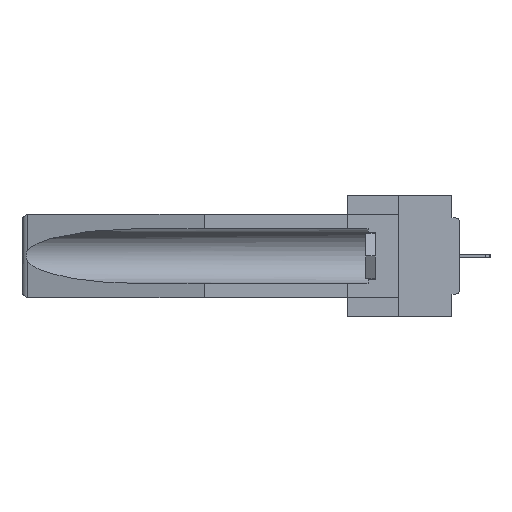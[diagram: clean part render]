
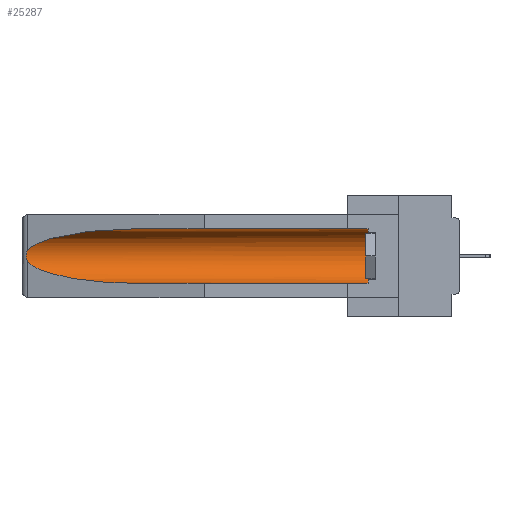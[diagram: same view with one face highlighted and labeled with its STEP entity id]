
A CAD part, left-side view. The second image highlights one B-rep face of the part: STEP entity #25287.
In plain terms, the highlighted cylindrical face has radius 2.857 mm (diameter 5.715 mm), a partial arc.
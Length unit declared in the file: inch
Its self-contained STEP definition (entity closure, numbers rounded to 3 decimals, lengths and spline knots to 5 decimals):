
#694 = FACE_OUTER_BOUND ( 'NONE', #26407, .T. ) ;
#1919 = VECTOR ( 'NONE', #34768, 39.37008 ) ;
#3051 = ORIENTED_EDGE ( 'NONE', *, *, #30657, .T. ) ;
#3149 = LINE ( 'NONE', #7410, #33691 ) ;
#3424 = CARTESIAN_POINT ( 'NONE',  ( 0.26537, 1.52718, -0.14972 ) ) ;
#5213 = CARTESIAN_POINT ( 'NONE',  ( 0.155, 1.07973, -0.059 ) ) ;
#5266 = CARTESIAN_POINT ( 'NONE',  ( 0.155, -0.30754, -0.284 ) ) ;
#5445 = CARTESIAN_POINT ( 'NONE',  ( 0.155, -0.30754, -0.1715 ) ) ;
#5881 = EDGE_CURVE ( 'NONE', #25886, #10236, #20941, .T. ) ;
#7076 = CARTESIAN_POINT ( 'NONE',  ( 0.155, 0.126, -0.1715 ) ) ;
#7410 = CARTESIAN_POINT ( 'NONE',  ( 0.155, -0.30754, -0.059 ) ) ;
#7877 = CYLINDRICAL_SURFACE ( 'NONE', #36250, 0.1125 ) ;
#7905 = DIRECTION ( 'NONE',  ( 0., 0., 1. ) ) ;
#9110 = CARTESIAN_POINT ( 'NONE',  ( 0.25451, 1.48313, -0.09465 ) ) ;
#9527 = CARTESIAN_POINT ( 'NONE',  ( 0.2673, 1.5327, -0.16383 ) ) ;
#10073 = DIRECTION ( 'NONE',  ( 0., 0., 1. ) ) ;
#10236 = VERTEX_POINT ( 'NONE', #14923 ) ;
#12125 = CARTESIAN_POINT ( 'NONE',  ( 0.155, 1.07973, -0.059 ) ) ;
#12360 = VERTEX_POINT ( 'NONE', #15434 ) ;
#12540 = CARTESIAN_POINT ( 'NONE',  ( 0.2675, 1.53308, -0.17534 ) ) ;
#13008 = CARTESIAN_POINT ( 'NONE',  ( 0.26537, 1.52718, -0.19328 ) ) ;
#13129 = CARTESIAN_POINT ( 'NONE',  ( 0.21114, 1.30732, -0.284 ) ) ;
#13159 = EDGE_CURVE ( 'NONE', #17250, #25886, #3149, .T. ) ;
#14923 = CARTESIAN_POINT ( 'NONE',  ( 0.26537, 1.52718, -0.14972 ) ) ;
#15116 = CARTESIAN_POINT ( 'NONE',  ( 0.26537, 1.52718, -0.14972 ) ) ;
#15328 = CARTESIAN_POINT ( 'NONE',  ( 0.26537, 1.52718, -0.19328 ) ) ;
#15434 = CARTESIAN_POINT ( 'NONE',  ( 0.155, 1.07973, -0.284 ) ) ;
#15507 = CARTESIAN_POINT ( 'NONE',  ( 0.26655, 1.53094, -0.18657 ) ) ;
#16606 = VERTEX_POINT ( 'NONE', #15328 ) ;
#16707 = EDGE_CURVE ( 'NONE', #16606, #12360, #22612, .T. ) ;
#16810 = ORIENTED_EDGE ( 'NONE', *, *, #37912, .F. ) ;
#17250 = VERTEX_POINT ( 'NONE', #36575 ) ;
#18498 = CARTESIAN_POINT ( 'NONE',  ( 0.26537, 1.52718, -0.19328 ) ) ;
#18957 = CARTESIAN_POINT ( 'NONE',  ( 0.25451, 1.48313, -0.24835 ) ) ;
#20941 =( BOUNDED_CURVE ( )  B_SPLINE_CURVE ( 3, ( #12125, #29770, #9110, #15116 ),
 .UNSPECIFIED., .F., .F. ) 
 B_SPLINE_CURVE_WITH_KNOTS ( ( 4, 4 ),
 ( 4.71239, 6.08839 ),
 .UNSPECIFIED. ) 
 CURVE ( )  GEOMETRIC_REPRESENTATION_ITEM ( )  RATIONAL_B_SPLINE_CURVE ( ( 1., 0.848, 0.848, 1. ) ) 
 REPRESENTATION_ITEM ( '' )  );
#21350 = CARTESIAN_POINT ( 'NONE',  ( 0.26597, 1.52961, -0.15275 ) ) ;
#21578 = B_SPLINE_CURVE_WITH_KNOTS ( 'NONE', 3,
 ( #3424, #21350, #27286, #9527, #30156, #12540, #33031, #15507, #35979, #18498 ),
 .UNSPECIFIED., .F., .F.,
 ( 4, 2, 2, 2, 4 ),
 ( 0., 0.00029, 0.00058, 0.00087, 0.00117 ),
 .UNSPECIFIED. ) ;
#22612 =( BOUNDED_CURVE ( )  B_SPLINE_CURVE ( 3, ( #13008, #18957, #13129, #33616 ),
 .UNSPECIFIED., .F., .F. ) 
 B_SPLINE_CURVE_WITH_KNOTS ( ( 4, 4 ),
 ( 0.1948, 1.5708 ),
 .UNSPECIFIED. ) 
 CURVE ( )  GEOMETRIC_REPRESENTATION_ITEM ( )  RATIONAL_B_SPLINE_CURVE ( ( 1., 0.848, 0.848, 1. ) ) 
 REPRESENTATION_ITEM ( '' )  );
#23614 = EDGE_CURVE ( 'NONE', #10236, #16606, #21578, .T. ) ;
#23621 = ORIENTED_EDGE ( 'NONE', *, *, #16707, .T. ) ;
#24448 = ORIENTED_EDGE ( 'NONE', *, *, #5881, .T. ) ;
#25287 = ADVANCED_FACE ( 'NONE', ( #694 ), #7877, .F. ) ;
#25886 = VERTEX_POINT ( 'NONE', #5213 ) ;
#26132 = CARTESIAN_POINT ( 'NONE',  ( 0.155, 0.126, -0.284 ) ) ;
#26407 = EDGE_LOOP ( 'NONE', ( #24448, #26884, #23621, #16810, #3051, #36839 ) ) ;
#26524 = CIRCLE ( 'NONE', #26577, 0.1125 ) ;
#26577 = AXIS2_PLACEMENT_3D ( 'NONE', #7076, #27825, #10073 ) ;
#26741 = LINE ( 'NONE', #5266, #1919 ) ;
#26884 = ORIENTED_EDGE ( 'NONE', *, *, #23614, .T. ) ;
#27286 = CARTESIAN_POINT ( 'NONE',  ( 0.26654, 1.53092, -0.15636 ) ) ;
#27825 = DIRECTION ( 'NONE',  ( 0., -1., 0. ) ) ;
#28161 = DIRECTION ( 'NONE',  ( 0., 1., 0. ) ) ;
#29770 = CARTESIAN_POINT ( 'NONE',  ( 0.21114, 1.30732, -0.059 ) ) ;
#30156 = CARTESIAN_POINT ( 'NONE',  ( 0.2675, 1.53308, -0.16763 ) ) ;
#30657 = EDGE_CURVE ( 'NONE', #31246, #17250, #26524, .T. ) ;
#31246 = VERTEX_POINT ( 'NONE', #26132 ) ;
#33031 = CARTESIAN_POINT ( 'NONE',  ( 0.2673, 1.53269, -0.17917 ) ) ;
#33616 = CARTESIAN_POINT ( 'NONE',  ( 0.155, 1.07973, -0.284 ) ) ;
#33691 = VECTOR ( 'NONE', #28161, 39.37008 ) ;
#34768 = DIRECTION ( 'NONE',  ( 0., 1., 0. ) ) ;
#35979 = CARTESIAN_POINT ( 'NONE',  ( 0.26597, 1.5296, -0.19026 ) ) ;
#36250 = AXIS2_PLACEMENT_3D ( 'NONE', #5445, #37747, #7905 ) ;
#36575 = CARTESIAN_POINT ( 'NONE',  ( 0.155, 0.126, -0.059 ) ) ;
#36839 = ORIENTED_EDGE ( 'NONE', *, *, #13159, .T. ) ;
#37747 = DIRECTION ( 'NONE',  ( 0., 1., 0. ) ) ;
#37912 = EDGE_CURVE ( 'NONE', #31246, #12360, #26741, .T. ) ;
